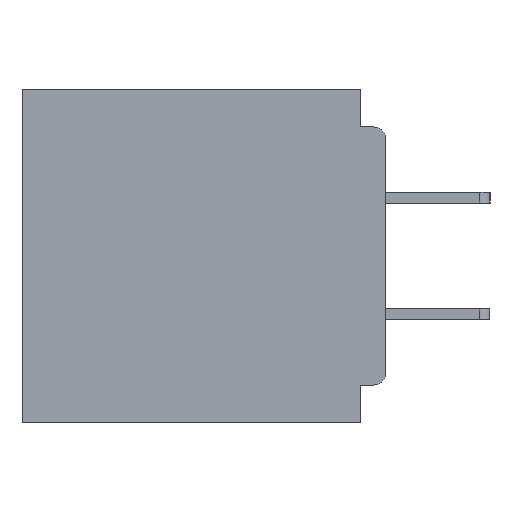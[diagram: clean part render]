
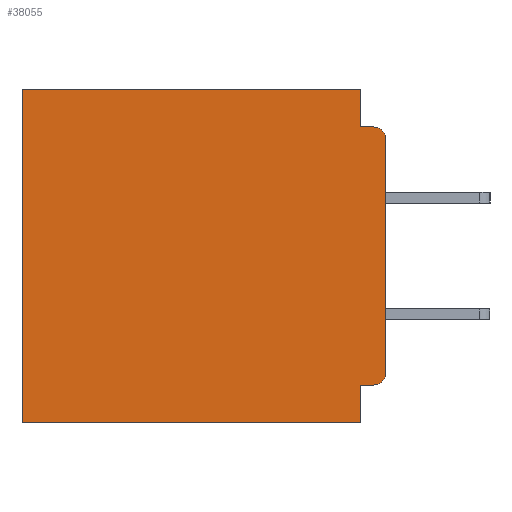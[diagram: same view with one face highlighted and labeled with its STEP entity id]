
A CAD part, left-side view. The second image highlights one B-rep face of the part: STEP entity #38055.
In plain terms, the highlighted planar face has unit normal (-1, 0, 0).
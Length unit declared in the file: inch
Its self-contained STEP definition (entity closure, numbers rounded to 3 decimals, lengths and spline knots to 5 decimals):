
#251 = AXIS2_PLACEMENT_3D ( 'NONE', #38769, #12367, #43187 ) ;
#2931 = VERTEX_POINT ( 'NONE', #11925 ) ;
#3140 = AXIS2_PLACEMENT_3D ( 'NONE', #32520, #6192, #36936 ) ;
#3989 = VERTEX_POINT ( 'NONE', #32990 ) ;
#4208 = FACE_OUTER_BOUND ( 'NONE', #37996, .T. ) ;
#5724 = PLANE ( 'NONE',  #19316 ) ;
#6192 = DIRECTION ( 'NONE',  ( -1., 0., 0. ) ) ;
#7145 = VECTOR ( 'NONE', #25083, 39.37008 ) ;
#7244 = CARTESIAN_POINT ( 'NONE',  ( 0.3, 0., -0.4 ) ) ;
#8087 = LINE ( 'NONE', #12683, #19738 ) ;
#8259 = LINE ( 'NONE', #14093, #31634 ) ;
#9064 = CARTESIAN_POINT ( 'NONE',  ( 0.3, 0.031, -0.355 ) ) ;
#9442 = EDGE_CURVE ( 'NONE', #28536, #3989, #17436, .T. ) ;
#10196 = CARTESIAN_POINT ( 'NONE',  ( 0.3, 0., -0.06 ) ) ;
#11793 = CARTESIAN_POINT ( 'NONE',  ( 0.3, 0.031, -0.045 ) ) ;
#11925 = CARTESIAN_POINT ( 'NONE',  ( 0.3, 0.031, 0. ) ) ;
#12045 = EDGE_CURVE ( 'NONE', #32945, #52734, #8259, .T. ) ;
#12367 = DIRECTION ( 'NONE',  ( -1., 0., 0. ) ) ;
#12475 = CARTESIAN_POINT ( 'NONE',  ( 0.3, 0.437, 0. ) ) ;
#12683 = CARTESIAN_POINT ( 'NONE',  ( 0.3, 0., 0. ) ) ;
#13805 = VECTOR ( 'NONE', #20262, 39.37008 ) ;
#14093 = CARTESIAN_POINT ( 'NONE',  ( 0.3, 0.031, -0.4 ) ) ;
#14564 = DIRECTION ( 'NONE',  ( 1., 0., 0. ) ) ;
#15205 = LINE ( 'NONE', #7244, #13805 ) ;
#15416 = VECTOR ( 'NONE', #35769, 39.37008 ) ;
#16215 = ORIENTED_EDGE ( 'NONE', *, *, #50274, .T. ) ;
#17436 = LINE ( 'NONE', #51594, #7145 ) ;
#19316 = AXIS2_PLACEMENT_3D ( 'NONE', #40978, #14564, #45431 ) ;
#19738 = VECTOR ( 'NONE', #43506, 39.37008 ) ;
#20262 = DIRECTION ( 'NONE',  ( 0., 1., 0. ) ) ;
#20449 = CARTESIAN_POINT ( 'NONE',  ( 0.3, 0.437, -0.4 ) ) ;
#20820 = ORIENTED_EDGE ( 'NONE', *, *, #32242, .F. ) ;
#21061 = ORIENTED_EDGE ( 'NONE', *, *, #33022, .F. ) ;
#21505 = VERTEX_POINT ( 'NONE', #12475 ) ;
#21649 = VECTOR ( 'NONE', #21940, 39.37008 ) ;
#21940 = DIRECTION ( 'NONE',  ( 0., 1., 0. ) ) ;
#22527 = ORIENTED_EDGE ( 'NONE', *, *, #30476, .F. ) ;
#24620 = VERTEX_POINT ( 'NONE', #10196 ) ;
#24768 = DIRECTION ( 'NONE',  ( 0., 0., -1. ) ) ;
#25083 = DIRECTION ( 'NONE',  ( 0., -1., 0. ) ) ;
#26149 = ORIENTED_EDGE ( 'NONE', *, *, #9442, .F. ) ;
#27081 = LINE ( 'NONE', #31337, #15416 ) ;
#28092 = CARTESIAN_POINT ( 'NONE',  ( 0.3, 0.031, -0.4 ) ) ;
#28514 = ORIENTED_EDGE ( 'NONE', *, *, #56893, .T. ) ;
#28536 = VERTEX_POINT ( 'NONE', #11793 ) ;
#29018 = VERTEX_POINT ( 'NONE', #32320 ) ;
#29460 = CARTESIAN_POINT ( 'NONE',  ( 0.3, 0., -0.34 ) ) ;
#29723 = LINE ( 'NONE', #49957, #51842 ) ;
#30476 = EDGE_CURVE ( 'NONE', #2931, #28536, #46818, .T. ) ;
#30969 = CIRCLE ( 'NONE', #3140, 0.015 ) ;
#31337 = CARTESIAN_POINT ( 'NONE',  ( 0.3, 0., -0.4 ) ) ;
#31634 = VECTOR ( 'NONE', #44946, 39.37008 ) ;
#32242 = EDGE_CURVE ( 'NONE', #29018, #32945, #47975, .T. ) ;
#32320 = CARTESIAN_POINT ( 'NONE',  ( 0.3, 0.015, -0.355 ) ) ;
#32520 = CARTESIAN_POINT ( 'NONE',  ( 0.3, 0.015, -0.34 ) ) ;
#32735 = CIRCLE ( 'NONE', #251, 0.015 ) ;
#32945 = VERTEX_POINT ( 'NONE', #9064 ) ;
#32990 = CARTESIAN_POINT ( 'NONE',  ( 0.3, 0.015, -0.045 ) ) ;
#33022 = EDGE_CURVE ( 'NONE', #24620, #54981, #27081, .T. ) ;
#34686 = EDGE_CURVE ( 'NONE', #2931, #21505, #8087, .T. ) ;
#34998 = VECTOR ( 'NONE', #24768, 39.37008 ) ;
#35769 = DIRECTION ( 'NONE',  ( 0., 0., -1. ) ) ;
#36344 = ORIENTED_EDGE ( 'NONE', *, *, #39312, .T. ) ;
#36570 = ORIENTED_EDGE ( 'NONE', *, *, #12045, .F. ) ;
#36936 = DIRECTION ( 'NONE',  ( 0., 0., -1. ) ) ;
#37996 = EDGE_LOOP ( 'NONE', ( #21061, #28514, #26149, #22527, #42480, #16215, #49631, #36570, #20820, #36344 ) ) ;
#38055 = ADVANCED_FACE ( 'NONE', ( #4208 ), #5724, .F. ) ;
#38301 = EDGE_CURVE ( 'NONE', #52734, #54022, #15205, .T. ) ;
#38769 = CARTESIAN_POINT ( 'NONE',  ( 0.3, 0.015, -0.06 ) ) ;
#39312 = EDGE_CURVE ( 'NONE', #29018, #54981, #30969, .T. ) ;
#40978 = CARTESIAN_POINT ( 'NONE',  ( 0.3, 0., -0.4 ) ) ;
#42480 = ORIENTED_EDGE ( 'NONE', *, *, #34686, .T. ) ;
#43187 = DIRECTION ( 'NONE',  ( 0., 0., -1. ) ) ;
#43506 = DIRECTION ( 'NONE',  ( 0., 1., 0. ) ) ;
#43993 = CARTESIAN_POINT ( 'NONE',  ( 0.3, 0., -0.355 ) ) ;
#44946 = DIRECTION ( 'NONE',  ( 0., 0., -1. ) ) ;
#45431 = DIRECTION ( 'NONE',  ( 0., 0., -1. ) ) ;
#46818 = LINE ( 'NONE', #46902, #34998 ) ;
#46902 = CARTESIAN_POINT ( 'NONE',  ( 0.3, 0.031, 0. ) ) ;
#47975 = LINE ( 'NONE', #43993, #21649 ) ;
#49631 = ORIENTED_EDGE ( 'NONE', *, *, #38301, .F. ) ;
#49957 = CARTESIAN_POINT ( 'NONE',  ( 0.3, 0.437, -0.4 ) ) ;
#50274 = EDGE_CURVE ( 'NONE', #21505, #54022, #29723, .T. ) ;
#51594 = CARTESIAN_POINT ( 'NONE',  ( 0.3, 0., -0.045 ) ) ;
#51842 = VECTOR ( 'NONE', #54336, 39.37008 ) ;
#52734 = VERTEX_POINT ( 'NONE', #28092 ) ;
#54022 = VERTEX_POINT ( 'NONE', #20449 ) ;
#54336 = DIRECTION ( 'NONE',  ( 0., 0., -1. ) ) ;
#54981 = VERTEX_POINT ( 'NONE', #29460 ) ;
#56893 = EDGE_CURVE ( 'NONE', #24620, #3989, #32735, .T. ) ;
